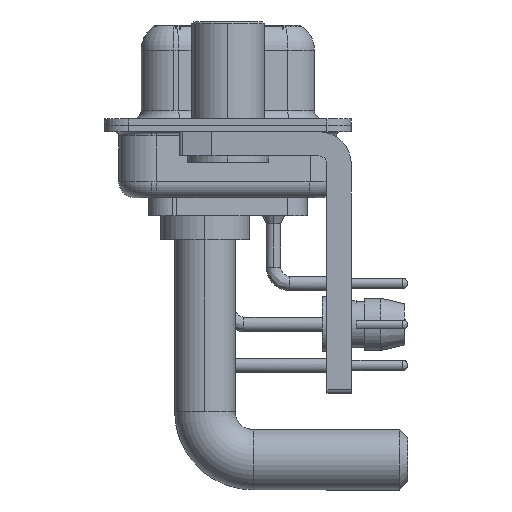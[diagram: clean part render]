
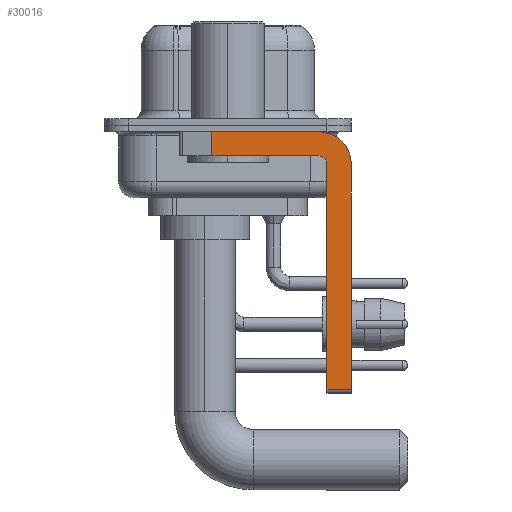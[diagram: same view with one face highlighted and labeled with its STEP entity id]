
A CAD part, left-side view. The second image highlights one B-rep face of the part: STEP entity #30016.
In plain terms, the highlighted planar face has unit normal (-1, 0, 0).
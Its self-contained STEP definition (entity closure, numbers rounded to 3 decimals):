
#195 = CIRCLE ( 'NONE', #29972, 2. ) ;
#1005 = CARTESIAN_POINT ( 'NONE',  ( -2.9, -7.65, -2.4 ) ) ;
#3079 = LINE ( 'NONE', #13725, #21301 ) ;
#5168 = DIRECTION ( 'NONE',  ( -1., 0., 0. ) ) ;
#5500 = EDGE_LOOP ( 'NONE', ( #9298, #26839, #29846, #17858, #32383, #20477, #18907, #17092 ) ) ;
#5714 = FACE_OUTER_BOUND ( 'NONE', #5500, .T. ) ;
#6320 = VERTEX_POINT ( 'NONE', #22794 ) ;
#6428 = LINE ( 'NONE', #1005, #29619 ) ;
#6622 = VERTEX_POINT ( 'NONE', #11566 ) ;
#7373 = CARTESIAN_POINT ( 'NONE',  ( -2.9, 0.978, -0.4 ) ) ;
#7769 = CARTESIAN_POINT ( 'NONE',  ( -2.9, -5.65, -1.9 ) ) ;
#8078 = DIRECTION ( 'NONE',  ( 0., 0., -1. ) ) ;
#8160 = DIRECTION ( 'NONE',  ( 0., 0., -1. ) ) ;
#8240 = EDGE_CURVE ( 'NONE', #24616, #15209, #3079, .T. ) ;
#9298 = ORIENTED_EDGE ( 'NONE', *, *, #21629, .F. ) ;
#10285 = LINE ( 'NONE', #7769, #29541 ) ;
#11037 = CARTESIAN_POINT ( 'NONE',  ( -2.9, -5.65, -2.4 ) ) ;
#11566 = CARTESIAN_POINT ( 'NONE',  ( -2.9, -6.15, -2.4 ) ) ;
#11651 = LINE ( 'NONE', #24237, #20932 ) ;
#11821 = DIRECTION ( 'NONE',  ( 0., 0., -1. ) ) ;
#12827 = DIRECTION ( 'NONE',  ( 0., 1., 0. ) ) ;
#13469 = DIRECTION ( 'NONE',  ( 1., 0., 0. ) ) ;
#13725 = CARTESIAN_POINT ( 'NONE',  ( -2.9, -5.65, -16.35 ) ) ;
#14190 = DIRECTION ( 'NONE',  ( 0., 0., -1. ) ) ;
#15209 = VERTEX_POINT ( 'NONE', #31063 ) ;
#15924 = DIRECTION ( 'NONE',  ( 1., 0., 0. ) ) ;
#16049 = DIRECTION ( 'NONE',  ( 0., -1., 0. ) ) ;
#17092 = ORIENTED_EDGE ( 'NONE', *, *, #26153, .F. ) ;
#17339 = EDGE_CURVE ( 'NONE', #22627, #15209, #6428, .T. ) ;
#17389 = EDGE_CURVE ( 'NONE', #22454, #32333, #11651, .T. ) ;
#17858 = ORIENTED_EDGE ( 'NONE', *, *, #19371, .F. ) ;
#18004 = EDGE_CURVE ( 'NONE', #24616, #6622, #20092, .T. ) ;
#18256 = AXIS2_PLACEMENT_3D ( 'NONE', #20580, #5168, #25355 ) ;
#18907 = ORIENTED_EDGE ( 'NONE', *, *, #17339, .F. ) ;
#19371 = EDGE_CURVE ( 'NONE', #6622, #6320, #27523, .T. ) ;
#19895 = CARTESIAN_POINT ( 'NONE',  ( -2.9, -5.65, -0.4 ) ) ;
#20092 = LINE ( 'NONE', #30446, #26928 ) ;
#20477 = ORIENTED_EDGE ( 'NONE', *, *, #8240, .T. ) ;
#20580 = CARTESIAN_POINT ( 'NONE',  ( -2.9, -5.65, -2.4 ) ) ;
#20932 = VECTOR ( 'NONE', #11821, 1000. ) ;
#21221 = CARTESIAN_POINT ( 'NONE',  ( -2.9, -6.15, -16.35 ) ) ;
#21301 = VECTOR ( 'NONE', #23439, 1000. ) ;
#21629 = EDGE_CURVE ( 'NONE', #22454, #24226, #26273, .T. ) ;
#21772 = CARTESIAN_POINT ( 'NONE',  ( -2.9, -7.65, -2.4 ) ) ;
#22454 = VERTEX_POINT ( 'NONE', #7373 ) ;
#22627 = VERTEX_POINT ( 'NONE', #21772 ) ;
#22794 = CARTESIAN_POINT ( 'NONE',  ( -2.9, -5.65, -1.9 ) ) ;
#23439 = DIRECTION ( 'NONE',  ( 0., -1., 0. ) ) ;
#23524 = PLANE ( 'NONE',  #25362 ) ;
#24226 = VERTEX_POINT ( 'NONE', #19895 ) ;
#24237 = CARTESIAN_POINT ( 'NONE',  ( -2.9, 0.978, -1.9 ) ) ;
#24616 = VERTEX_POINT ( 'NONE', #21221 ) ;
#25355 = DIRECTION ( 'NONE',  ( 0., 0., 1. ) ) ;
#25362 = AXIS2_PLACEMENT_3D ( 'NONE', #28769, #13469, #8078 ) ;
#26153 = EDGE_CURVE ( 'NONE', #24226, #22627, #195, .T. ) ;
#26273 = LINE ( 'NONE', #31032, #31944 ) ;
#26839 = ORIENTED_EDGE ( 'NONE', *, *, #17389, .T. ) ;
#26928 = VECTOR ( 'NONE', #27907, 1000. ) ;
#27110 = EDGE_CURVE ( 'NONE', #6320, #32333, #10285, .T. ) ;
#27523 = CIRCLE ( 'NONE', #18256, 0.5 ) ;
#27907 = DIRECTION ( 'NONE',  ( 0., 0., 1. ) ) ;
#28769 = CARTESIAN_POINT ( 'NONE',  ( -2.9, -5.65, -2.4 ) ) ;
#29541 = VECTOR ( 'NONE', #12827, 1000. ) ;
#29619 = VECTOR ( 'NONE', #14190, 1000. ) ;
#29846 = ORIENTED_EDGE ( 'NONE', *, *, #27110, .F. ) ;
#29972 = AXIS2_PLACEMENT_3D ( 'NONE', #11037, #15924, #8160 ) ;
#30016 = ADVANCED_FACE ( 'NONE', ( #5714 ), #23524, .F. ) ;
#30446 = CARTESIAN_POINT ( 'NONE',  ( -2.9, -6.15, -16.6 ) ) ;
#31032 = CARTESIAN_POINT ( 'NONE',  ( -2.9, 3., -0.4 ) ) ;
#31063 = CARTESIAN_POINT ( 'NONE',  ( -2.9, -7.65, -16.35 ) ) ;
#31077 = CARTESIAN_POINT ( 'NONE',  ( -2.9, 0.978, -1.9 ) ) ;
#31944 = VECTOR ( 'NONE', #16049, 1000. ) ;
#32333 = VERTEX_POINT ( 'NONE', #31077 ) ;
#32383 = ORIENTED_EDGE ( 'NONE', *, *, #18004, .F. ) ;
